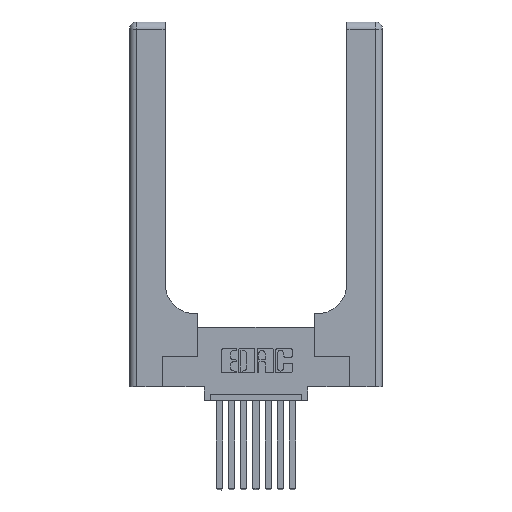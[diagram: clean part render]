
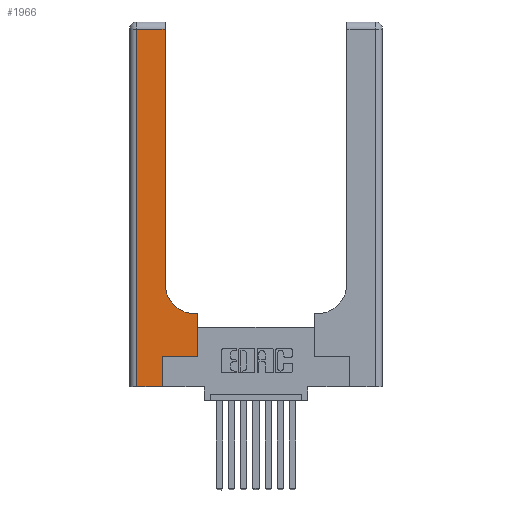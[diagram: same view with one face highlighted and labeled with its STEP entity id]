
A CAD part, top view. The second image highlights one B-rep face of the part: STEP entity #1966.
In plain terms, the highlighted planar face has unit normal (0, 0, 1).
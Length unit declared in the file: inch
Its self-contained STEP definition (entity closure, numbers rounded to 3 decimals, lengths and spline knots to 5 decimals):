
#385 = CARTESIAN_POINT ( 'NONE',  ( 0.269, 0.25, 0.37 ) ) ;
#666 = CARTESIAN_POINT ( 'NONE',  ( 0.269, 0., 0.37 ) ) ;
#803 = VERTEX_POINT ( 'NONE', #6073 ) ;
#813 = VECTOR ( 'NONE', #14661, 39.37008 ) ;
#824 = DIRECTION ( 'NONE',  ( -1., 0., 0. ) ) ;
#1012 = EDGE_CURVE ( 'NONE', #6671, #3575, #14502, .T. ) ;
#1866 = VECTOR ( 'NONE', #14309, 39.37008 ) ;
#1874 = CARTESIAN_POINT ( 'NONE',  ( 0., 2.94, 0.37 ) ) ;
#1966 = ADVANCED_FACE ( 'NONE', ( #6291 ), #12206, .F. ) ;
#2005 = LINE ( 'NONE', #9199, #4232 ) ;
#2202 = DIRECTION ( 'NONE',  ( 1., 0., 0. ) ) ;
#2344 = DIRECTION ( 'NONE',  ( 0., 1., 0. ) ) ;
#2416 = EDGE_LOOP ( 'NONE', ( #8847, #9885, #13184, #4156, #3943, #14495, #10586, #10137, #8253 ) ) ;
#2480 = VERTEX_POINT ( 'NONE', #12338 ) ;
#2511 = CARTESIAN_POINT ( 'NONE',  ( 0.2915, 0.6, 0.37 ) ) ;
#2815 = EDGE_CURVE ( 'NONE', #8089, #6671, #6275, .T. ) ;
#2935 = VERTEX_POINT ( 'NONE', #385 ) ;
#3036 = VECTOR ( 'NONE', #2202, 39.37008 ) ;
#3243 = VECTOR ( 'NONE', #2344, 39.37008 ) ;
#3416 = DIRECTION ( 'NONE',  ( 0., 1., 0. ) ) ;
#3575 = VERTEX_POINT ( 'NONE', #666 ) ;
#3824 = AXIS2_PLACEMENT_3D ( 'NONE', #13813, #8095, #6887 ) ;
#3943 = ORIENTED_EDGE ( 'NONE', *, *, #7737, .T. ) ;
#4156 = ORIENTED_EDGE ( 'NONE', *, *, #1012, .T. ) ;
#4232 = VECTOR ( 'NONE', #4475, 39.37008 ) ;
#4475 = DIRECTION ( 'NONE',  ( 1., 0., 0. ) ) ;
#4589 = CARTESIAN_POINT ( 'NONE',  ( 0.5585, 0.25, 0.37 ) ) ;
#4609 = EDGE_CURVE ( 'NONE', #2935, #14994, #2005, .T. ) ;
#6073 = CARTESIAN_POINT ( 'NONE',  ( 0.2915, 2.94, 0.37 ) ) ;
#6211 = VERTEX_POINT ( 'NONE', #7663 ) ;
#6275 = LINE ( 'NONE', #13550, #813 ) ;
#6291 = FACE_OUTER_BOUND ( 'NONE', #2416, .T. ) ;
#6387 = DIRECTION ( 'NONE',  ( 0., 1., 0. ) ) ;
#6671 = VERTEX_POINT ( 'NONE', #6994 ) ;
#6887 = DIRECTION ( 'NONE',  ( 1., 0., 0. ) ) ;
#6994 = CARTESIAN_POINT ( 'NONE',  ( 0.06, 0., 0.37 ) ) ;
#7163 = VECTOR ( 'NONE', #824, 39.37008 ) ;
#7247 = EDGE_CURVE ( 'NONE', #14994, #6211, #10163, .T. ) ;
#7663 = CARTESIAN_POINT ( 'NONE',  ( 0.5585, 0.6, 0.37 ) ) ;
#7737 = EDGE_CURVE ( 'NONE', #3575, #2935, #12613, .T. ) ;
#8071 = LINE ( 'NONE', #1874, #7163 ) ;
#8089 = VERTEX_POINT ( 'NONE', #13232 ) ;
#8095 = DIRECTION ( 'NONE',  ( 0., 0., -1. ) ) ;
#8253 = ORIENTED_EDGE ( 'NONE', *, *, #9573, .T. ) ;
#8314 = EDGE_CURVE ( 'NONE', #10197, #803, #8544, .T. ) ;
#8544 = LINE ( 'NONE', #11129, #9830 ) ;
#8847 = ORIENTED_EDGE ( 'NONE', *, *, #8314, .T. ) ;
#9182 = CARTESIAN_POINT ( 'NONE',  ( 0., 0., 0.37 ) ) ;
#9199 = CARTESIAN_POINT ( 'NONE',  ( 0.269, 0.25, 0.37 ) ) ;
#9303 = CARTESIAN_POINT ( 'NONE',  ( 0.5585, 0.25, 0.37 ) ) ;
#9573 = EDGE_CURVE ( 'NONE', #2480, #10197, #14944, .T. ) ;
#9830 = VECTOR ( 'NONE', #3416, 39.37008 ) ;
#9885 = ORIENTED_EDGE ( 'NONE', *, *, #13720, .T. ) ;
#10137 = ORIENTED_EDGE ( 'NONE', *, *, #12705, .T. ) ;
#10163 = LINE ( 'NONE', #9303, #3243 ) ;
#10197 = VERTEX_POINT ( 'NONE', #11853 ) ;
#10586 = ORIENTED_EDGE ( 'NONE', *, *, #7247, .T. ) ;
#10632 = CARTESIAN_POINT ( 'NONE',  ( 0.269, 0., 0.37 ) ) ;
#10920 = DIRECTION ( 'NONE',  ( -1., 0., 0. ) ) ;
#11129 = CARTESIAN_POINT ( 'NONE',  ( 0.2915, 3., 0.37 ) ) ;
#11732 = LINE ( 'NONE', #2511, #1866 ) ;
#11853 = CARTESIAN_POINT ( 'NONE',  ( 0.2915, 0.85, 0.37 ) ) ;
#12206 = PLANE ( 'NONE',  #13601 ) ;
#12338 = CARTESIAN_POINT ( 'NONE',  ( 0.5415, 0.6, 0.37 ) ) ;
#12613 = LINE ( 'NONE', #10632, #14607 ) ;
#12705 = EDGE_CURVE ( 'NONE', #6211, #2480, #11732, .T. ) ;
#13184 = ORIENTED_EDGE ( 'NONE', *, *, #2815, .T. ) ;
#13232 = CARTESIAN_POINT ( 'NONE',  ( 0.06, 2.94, 0.37 ) ) ;
#13376 = CARTESIAN_POINT ( 'NONE',  ( 0., 3., 0.37 ) ) ;
#13550 = CARTESIAN_POINT ( 'NONE',  ( 0.06, 3., 0.37 ) ) ;
#13601 = AXIS2_PLACEMENT_3D ( 'NONE', #13376, #14538, #10920 ) ;
#13720 = EDGE_CURVE ( 'NONE', #803, #8089, #8071, .T. ) ;
#13813 = CARTESIAN_POINT ( 'NONE',  ( 0.5415, 0.85, 0.37 ) ) ;
#14309 = DIRECTION ( 'NONE',  ( -1., 0., 0. ) ) ;
#14495 = ORIENTED_EDGE ( 'NONE', *, *, #4609, .T. ) ;
#14502 = LINE ( 'NONE', #9182, #3036 ) ;
#14538 = DIRECTION ( 'NONE',  ( 0., 0., -1. ) ) ;
#14607 = VECTOR ( 'NONE', #6387, 39.37008 ) ;
#14661 = DIRECTION ( 'NONE',  ( 0., -1., 0. ) ) ;
#14944 = CIRCLE ( 'NONE', #3824, 0.25 ) ;
#14994 = VERTEX_POINT ( 'NONE', #4589 ) ;
